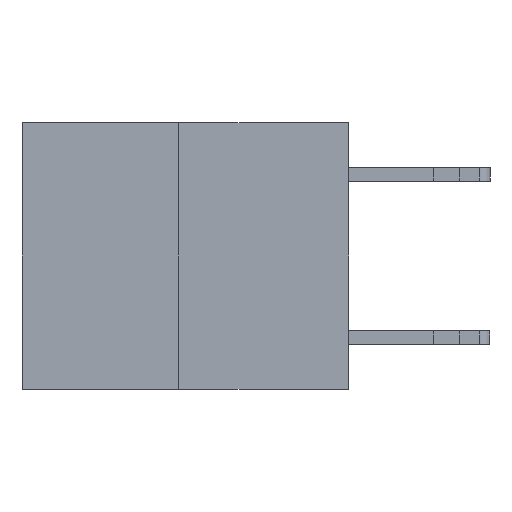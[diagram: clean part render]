
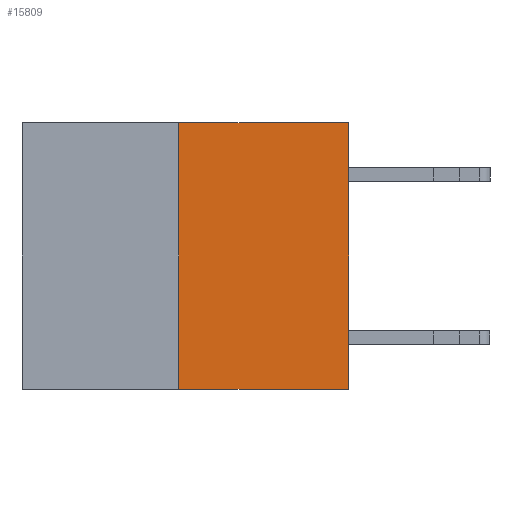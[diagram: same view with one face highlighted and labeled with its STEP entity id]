
A CAD part, left-side view. The second image highlights one B-rep face of the part: STEP entity #15809.
In plain terms, the highlighted planar face has unit normal (-1, 0, 0).
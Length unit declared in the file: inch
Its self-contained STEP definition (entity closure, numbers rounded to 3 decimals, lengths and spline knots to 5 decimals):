
#41 = ORIENTED_EDGE ( 'NONE', *, *, #5773, .F. ) ;
#89 = VECTOR ( 'NONE', #18436, 39.37008 ) ;
#1183 = DIRECTION ( 'NONE',  ( 0., -1., 0. ) ) ;
#1589 = ORIENTED_EDGE ( 'NONE', *, *, #8352, .F. ) ;
#1740 = LINE ( 'NONE', #9894, #8085 ) ;
#2446 = CARTESIAN_POINT ( 'NONE',  ( 0., 0.6, 0. ) ) ;
#3502 = VECTOR ( 'NONE', #1183, 39.37008 ) ;
#3631 = DIRECTION ( 'NONE',  ( 0., 0., -1. ) ) ;
#3882 = PLANE ( 'NONE',  #9448 ) ;
#4072 = LINE ( 'NONE', #11958, #89 ) ;
#4712 = CARTESIAN_POINT ( 'NONE',  ( 0., 0., 0. ) ) ;
#5205 = DIRECTION ( 'NONE',  ( 0., -1., 0. ) ) ;
#5773 = EDGE_CURVE ( 'NONE', #6758, #10846, #4072, .T. ) ;
#5975 = EDGE_CURVE ( 'NONE', #6758, #12010, #1740, .T. ) ;
#6758 = VERTEX_POINT ( 'NONE', #14000 ) ;
#6830 = VECTOR ( 'NONE', #10836, 39.37008 ) ;
#7810 = EDGE_CURVE ( 'NONE', #12010, #17263, #15972, .T. ) ;
#8085 = VECTOR ( 'NONE', #5205, 39.37008 ) ;
#8221 = DIRECTION ( 'NONE',  ( 1., 0., 0. ) ) ;
#8352 = EDGE_CURVE ( 'NONE', #10846, #17263, #11737, .T. ) ;
#8729 = EDGE_LOOP ( 'NONE', ( #41, #14150, #19271, #1589 ) ) ;
#9448 = AXIS2_PLACEMENT_3D ( 'NONE', #2446, #8221, #3631 ) ;
#9894 = CARTESIAN_POINT ( 'NONE',  ( 0., 0.6, -0.49 ) ) ;
#10341 = CARTESIAN_POINT ( 'NONE',  ( 0., 0., -0.49 ) ) ;
#10836 = DIRECTION ( 'NONE',  ( 0., 0., 1. ) ) ;
#10846 = VERTEX_POINT ( 'NONE', #13772 ) ;
#11737 = LINE ( 'NONE', #14619, #3502 ) ;
#11958 = CARTESIAN_POINT ( 'NONE',  ( 0., 0.312, -0.49 ) ) ;
#12010 = VERTEX_POINT ( 'NONE', #10341 ) ;
#13570 = CARTESIAN_POINT ( 'NONE',  ( 0., 0., 0. ) ) ;
#13772 = CARTESIAN_POINT ( 'NONE',  ( 0., 0.312, 0. ) ) ;
#14000 = CARTESIAN_POINT ( 'NONE',  ( 0., 0.312, -0.49 ) ) ;
#14150 = ORIENTED_EDGE ( 'NONE', *, *, #5975, .T. ) ;
#14619 = CARTESIAN_POINT ( 'NONE',  ( 0., 0.6, 0. ) ) ;
#15809 = ADVANCED_FACE ( 'NONE', ( #19067 ), #3882, .F. ) ;
#15972 = LINE ( 'NONE', #4712, #6830 ) ;
#17263 = VERTEX_POINT ( 'NONE', #13570 ) ;
#18436 = DIRECTION ( 'NONE',  ( 0., 0., 1. ) ) ;
#19067 = FACE_OUTER_BOUND ( 'NONE', #8729, .T. ) ;
#19271 = ORIENTED_EDGE ( 'NONE', *, *, #7810, .T. ) ;
